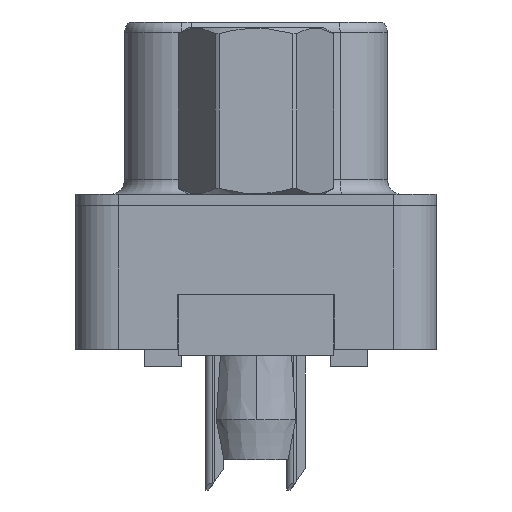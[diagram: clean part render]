
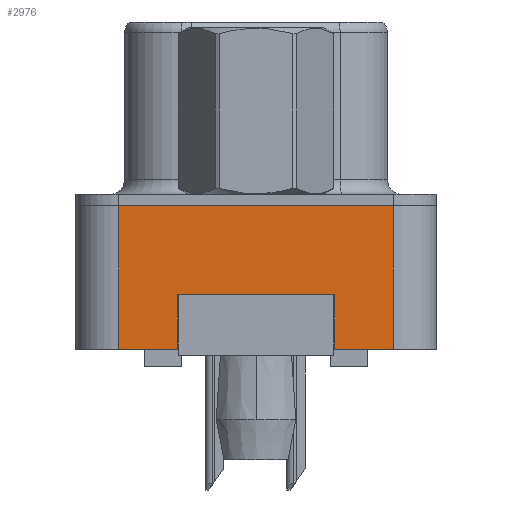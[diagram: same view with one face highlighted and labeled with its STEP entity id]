
A CAD part, left-side view. The second image highlights one B-rep face of the part: STEP entity #2976.
In plain terms, the highlighted planar face has unit normal (-1, 0, 0).
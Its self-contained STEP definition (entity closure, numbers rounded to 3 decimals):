
#545 = EDGE_CURVE ( 'NONE', #5417, #21718, #16723, .T. ) ;
#608 = CARTESIAN_POINT ( 'NONE',  ( -3., 2.75, -3.1 ) ) ;
#936 = LINE ( 'NONE', #9496, #22241 ) ;
#1183 = VERTEX_POINT ( 'NONE', #27443 ) ;
#1942 = ORIENTED_EDGE ( 'NONE', *, *, #24736, .T. ) ;
#2276 = PLANE ( 'NONE',  #3862 ) ;
#2837 = ORIENTED_EDGE ( 'NONE', *, *, #21076, .F. ) ;
#2976 = ADVANCED_FACE ( 'NONE', ( #13251 ), #2276, .T. ) ;
#3336 = VECTOR ( 'NONE', #23372, 1000. ) ;
#3342 = VECTOR ( 'NONE', #23578, 1000. ) ;
#3435 = CARTESIAN_POINT ( 'NONE',  ( -3., -4.775, -5. ) ) ;
#3862 = AXIS2_PLACEMENT_3D ( 'NONE', #10987, #19474, #21883 ) ;
#4416 = VECTOR ( 'NONE', #15681, 1000. ) ;
#5409 = LINE ( 'NONE', #20682, #10740 ) ;
#5417 = VERTEX_POINT ( 'NONE', #24628 ) ;
#5784 = LINE ( 'NONE', #21054, #3342 ) ;
#6227 = LINE ( 'NONE', #25865, #13045 ) ;
#6327 = ORIENTED_EDGE ( 'NONE', *, *, #9797, .T. ) ;
#8680 = CARTESIAN_POINT ( 'NONE',  ( -3., -4.775, -5. ) ) ;
#9496 = CARTESIAN_POINT ( 'NONE',  ( -3., 4.775, -5. ) ) ;
#9677 = VERTEX_POINT ( 'NONE', #3435 ) ;
#9713 = ORIENTED_EDGE ( 'NONE', *, *, #545, .F. ) ;
#9797 = EDGE_CURVE ( 'NONE', #22558, #11935, #6227, .T. ) ;
#10546 = VECTOR ( 'NONE', #17175, 1000. ) ;
#10740 = VECTOR ( 'NONE', #14012, 1000. ) ;
#10849 = VERTEX_POINT ( 'NONE', #608 ) ;
#10987 = CARTESIAN_POINT ( 'NONE',  ( -3., -4.775, -5. ) ) ;
#11935 = VERTEX_POINT ( 'NONE', #17781 ) ;
#13045 = VECTOR ( 'NONE', #14704, 1000. ) ;
#13251 = FACE_OUTER_BOUND ( 'NONE', #16054, .T. ) ;
#13404 = CARTESIAN_POINT ( 'NONE',  ( -3., 2.75, -3.1 ) ) ;
#14012 = DIRECTION ( 'NONE',  ( 0., 1., 0. ) ) ;
#14130 = EDGE_CURVE ( 'NONE', #22558, #5417, #936, .T. ) ;
#14704 = DIRECTION ( 'NONE',  ( 0., -1., 0. ) ) ;
#14777 = LINE ( 'NONE', #19299, #26614 ) ;
#15167 = VERTEX_POINT ( 'NONE', #22887 ) ;
#15334 = LINE ( 'NONE', #8680, #10546 ) ;
#15547 = LINE ( 'NONE', #13404, #4416 ) ;
#15681 = DIRECTION ( 'NONE',  ( 0., 0., -1. ) ) ;
#16054 = EDGE_LOOP ( 'NONE', ( #18435, #16605, #1942, #9713, #26529, #6327, #2837, #27588 ) ) ;
#16296 = EDGE_CURVE ( 'NONE', #1183, #15167, #5784, .T. ) ;
#16605 = ORIENTED_EDGE ( 'NONE', *, *, #16957, .T. ) ;
#16723 = LINE ( 'NONE', #23509, #3336 ) ;
#16957 = EDGE_CURVE ( 'NONE', #15167, #9677, #15334, .T. ) ;
#17048 = DIRECTION ( 'NONE',  ( 0., 0., 1. ) ) ;
#17175 = DIRECTION ( 'NONE',  ( 0., -1., 0. ) ) ;
#17690 = CARTESIAN_POINT ( 'NONE',  ( -3., -4.775, 0. ) ) ;
#17781 = CARTESIAN_POINT ( 'NONE',  ( -3., 2.75, -5. ) ) ;
#18435 = ORIENTED_EDGE ( 'NONE', *, *, #16296, .T. ) ;
#19299 = CARTESIAN_POINT ( 'NONE',  ( -3., -4.775, -5. ) ) ;
#19474 = DIRECTION ( 'NONE',  ( -1., 0., 0. ) ) ;
#20682 = CARTESIAN_POINT ( 'NONE',  ( -3., 2.75, -3.1 ) ) ;
#21054 = CARTESIAN_POINT ( 'NONE',  ( -3., -2.75, -3.1 ) ) ;
#21076 = EDGE_CURVE ( 'NONE', #10849, #11935, #15547, .T. ) ;
#21718 = VERTEX_POINT ( 'NONE', #17690 ) ;
#21883 = DIRECTION ( 'NONE',  ( 0., 0., 1. ) ) ;
#22241 = VECTOR ( 'NONE', #22528, 1000. ) ;
#22528 = DIRECTION ( 'NONE',  ( 0., 0., 1. ) ) ;
#22558 = VERTEX_POINT ( 'NONE', #23990 ) ;
#22887 = CARTESIAN_POINT ( 'NONE',  ( -3., -2.75, -5. ) ) ;
#23183 = EDGE_CURVE ( 'NONE', #1183, #10849, #5409, .T. ) ;
#23372 = DIRECTION ( 'NONE',  ( 0., -1., 0. ) ) ;
#23509 = CARTESIAN_POINT ( 'NONE',  ( -3., -4.775, 0. ) ) ;
#23578 = DIRECTION ( 'NONE',  ( 0., 0., -1. ) ) ;
#23990 = CARTESIAN_POINT ( 'NONE',  ( -3., 4.775, -5. ) ) ;
#24628 = CARTESIAN_POINT ( 'NONE',  ( -3., 4.775, 0. ) ) ;
#24736 = EDGE_CURVE ( 'NONE', #9677, #21718, #14777, .T. ) ;
#25865 = CARTESIAN_POINT ( 'NONE',  ( -3., -4.775, -5. ) ) ;
#26529 = ORIENTED_EDGE ( 'NONE', *, *, #14130, .F. ) ;
#26614 = VECTOR ( 'NONE', #17048, 1000. ) ;
#27443 = CARTESIAN_POINT ( 'NONE',  ( -3., -2.75, -3.1 ) ) ;
#27588 = ORIENTED_EDGE ( 'NONE', *, *, #23183, .F. ) ;
